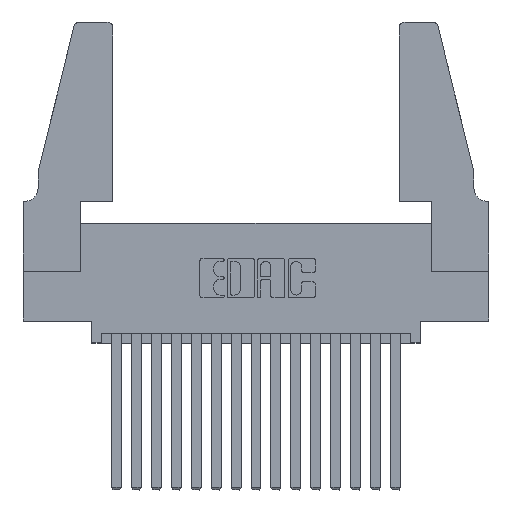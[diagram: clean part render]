
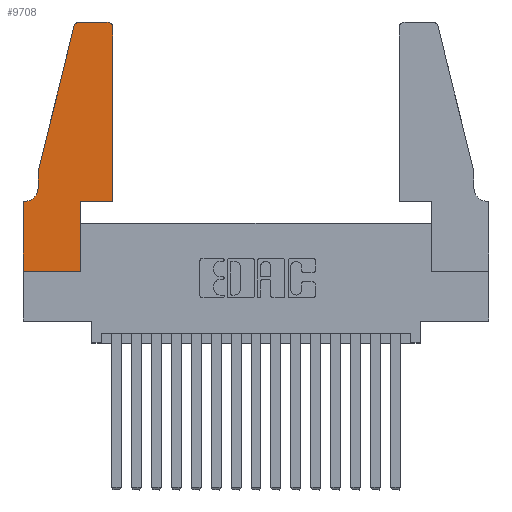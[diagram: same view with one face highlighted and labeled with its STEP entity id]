
A CAD part, top view. The second image highlights one B-rep face of the part: STEP entity #9708.
In plain terms, the highlighted planar face has unit normal (0, 0, 1).
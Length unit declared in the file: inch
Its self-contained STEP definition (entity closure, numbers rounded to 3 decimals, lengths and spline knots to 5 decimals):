
#396 = VECTOR ( 'NONE', #13454, 39.37008 ) ;
#656 = DIRECTION ( 'NONE',  ( 1., 0., 0. ) ) ;
#719 = VECTOR ( 'NONE', #10200, 39.37008 ) ;
#745 = PLANE ( 'NONE',  #5814 ) ;
#1059 = ORIENTED_EDGE ( 'NONE', *, *, #10012, .T. ) ;
#1159 = VERTEX_POINT ( 'NONE', #11331 ) ;
#1161 = LINE ( 'NONE', #16680, #719 ) ;
#1194 = LINE ( 'NONE', #2039, #4516 ) ;
#1454 = VERTEX_POINT ( 'NONE', #4281 ) ;
#1614 = VERTEX_POINT ( 'NONE', #7351 ) ;
#1761 = AXIS2_PLACEMENT_3D ( 'NONE', #14737, #6851, #16044 ) ;
#1959 = VECTOR ( 'NONE', #5132, 39.37008 ) ;
#2039 = CARTESIAN_POINT ( 'NONE',  ( 0.0755, 0.5, 0.37 ) ) ;
#2052 = LINE ( 'NONE', #10939, #9015 ) ;
#2414 = LINE ( 'NONE', #14403, #1959 ) ;
#2603 = EDGE_CURVE ( 'NONE', #14687, #13880, #5997, .T. ) ;
#2638 = CARTESIAN_POINT ( 'NONE',  ( 0.0755, 0.42, 0.37 ) ) ;
#3255 = AXIS2_PLACEMENT_3D ( 'NONE', #16836, #9037, #656 ) ;
#3266 = AXIS2_PLACEMENT_3D ( 'NONE', #7038, #16215, #8405 ) ;
#3308 = ORIENTED_EDGE ( 'NONE', *, *, #16690, .T. ) ;
#3374 = LINE ( 'NONE', #16887, #6653 ) ;
#3428 = VERTEX_POINT ( 'NONE', #11575 ) ;
#3618 = DIRECTION ( 'NONE',  ( 0., 0., 1. ) ) ;
#3692 = EDGE_CURVE ( 'NONE', #13880, #1159, #12225, .T. ) ;
#3773 = LINE ( 'NONE', #17414, #17524 ) ;
#4142 = DIRECTION ( 'NONE',  ( -1., 0., 0. ) ) ;
#4281 = CARTESIAN_POINT ( 'NONE',  ( 0., 0.35, 0.37 ) ) ;
#4516 = VECTOR ( 'NONE', #15460, 39.37008 ) ;
#5132 = DIRECTION ( 'NONE',  ( 0., 1., 0. ) ) ;
#5319 = VERTEX_POINT ( 'NONE', #12757 ) ;
#5472 = CARTESIAN_POINT ( 'NONE',  ( 0.2605, 1.25, 0.37 ) ) ;
#5486 = LINE ( 'NONE', #8207, #396 ) ;
#5509 = EDGE_CURVE ( 'NONE', #14080, #11525, #2414, .T. ) ;
#5814 = AXIS2_PLACEMENT_3D ( 'NONE', #11748, #3618, #13016 ) ;
#5864 = CARTESIAN_POINT ( 'NONE',  ( 0.0755, 0.5, 0.37 ) ) ;
#5997 = LINE ( 'NONE', #6854, #16541 ) ;
#6073 = VECTOR ( 'NONE', #12280, 39.37008 ) ;
#6595 = ORIENTED_EDGE ( 'NONE', *, *, #5509, .T. ) ;
#6653 = VECTOR ( 'NONE', #10412, 39.37008 ) ;
#6851 = DIRECTION ( 'NONE',  ( 0., 0., -1. ) ) ;
#6854 = CARTESIAN_POINT ( 'NONE',  ( 0.0755, 0.5, 0.37 ) ) ;
#7038 = CARTESIAN_POINT ( 'NONE',  ( 0.4205, 1.22, 0.37 ) ) ;
#7351 = CARTESIAN_POINT ( 'NONE',  ( 0.25487, 1.22718, 0.37 ) ) ;
#8207 = CARTESIAN_POINT ( 'NONE',  ( 0.4505, 0.35, 0.37 ) ) ;
#8274 = DIRECTION ( 'NONE',  ( 1., 0., 0. ) ) ;
#8376 = DIRECTION ( 'NONE',  ( 0., -1., 0. ) ) ;
#8405 = DIRECTION ( 'NONE',  ( 1., 0., 0. ) ) ;
#8479 = EDGE_CURVE ( 'NONE', #14214, #3428, #17027, .T. ) ;
#9015 = VECTOR ( 'NONE', #4142, 39.37008 ) ;
#9037 = DIRECTION ( 'NONE',  ( 0., 0., 1. ) ) ;
#9352 = ORIENTED_EDGE ( 'NONE', *, *, #9587, .T. ) ;
#9482 = VERTEX_POINT ( 'NONE', #14347 ) ;
#9537 = ORIENTED_EDGE ( 'NONE', *, *, #8479, .T. ) ;
#9587 = EDGE_CURVE ( 'NONE', #1454, #11561, #1161, .T. ) ;
#9708 = ADVANCED_FACE ( 'NONE', ( #16142 ), #745, .T. ) ;
#10012 = EDGE_CURVE ( 'NONE', #1159, #1454, #2052, .T. ) ;
#10200 = DIRECTION ( 'NONE',  ( 0., -1., 0. ) ) ;
#10270 = CARTESIAN_POINT ( 'NONE',  ( 0.2865, 0.35, 0.37 ) ) ;
#10324 = EDGE_CURVE ( 'NONE', #3428, #1614, #14487, .T. ) ;
#10359 = EDGE_CURVE ( 'NONE', #5319, #9482, #3374, .T. ) ;
#10381 = CARTESIAN_POINT ( 'NONE',  ( 0., 0., 0.37 ) ) ;
#10412 = DIRECTION ( 'NONE',  ( 0., 1., 0. ) ) ;
#10585 = ORIENTED_EDGE ( 'NONE', *, *, #10359, .T. ) ;
#10939 = CARTESIAN_POINT ( 'NONE',  ( 0.0755, 0.35, 0.37 ) ) ;
#11192 = ORIENTED_EDGE ( 'NONE', *, *, #13065, .T. ) ;
#11305 = CARTESIAN_POINT ( 'NONE',  ( 0.2865, 0., 0.37 ) ) ;
#11331 = CARTESIAN_POINT ( 'NONE',  ( 0.0055, 0.35, 0.37 ) ) ;
#11525 = VERTEX_POINT ( 'NONE', #10270 ) ;
#11561 = VERTEX_POINT ( 'NONE', #10381 ) ;
#11575 = CARTESIAN_POINT ( 'NONE',  ( 0.284, 1.25, 0.37 ) ) ;
#11748 = CARTESIAN_POINT ( 'NONE',  ( 0., 0.35, 0.37 ) ) ;
#11823 = EDGE_CURVE ( 'NONE', #11561, #14080, #3773, .T. ) ;
#12225 = CIRCLE ( 'NONE', #1761, 0.07 ) ;
#12280 = DIRECTION ( 'NONE',  ( -1., 0., 0. ) ) ;
#12757 = CARTESIAN_POINT ( 'NONE',  ( 0.4505, 0.35, 0.37 ) ) ;
#12797 = CIRCLE ( 'NONE', #3266, 0.03 ) ;
#13016 = DIRECTION ( 'NONE',  ( 1., 0., 0. ) ) ;
#13065 = EDGE_CURVE ( 'NONE', #1614, #14687, #1194, .T. ) ;
#13454 = DIRECTION ( 'NONE',  ( 1., 0., 0. ) ) ;
#13810 = ORIENTED_EDGE ( 'NONE', *, *, #10324, .T. ) ;
#13880 = VERTEX_POINT ( 'NONE', #2638 ) ;
#14080 = VERTEX_POINT ( 'NONE', #11305 ) ;
#14111 = CARTESIAN_POINT ( 'NONE',  ( 0.4205, 1.25, 0.37 ) ) ;
#14214 = VERTEX_POINT ( 'NONE', #14111 ) ;
#14347 = CARTESIAN_POINT ( 'NONE',  ( 0.4505, 1.22, 0.37 ) ) ;
#14403 = CARTESIAN_POINT ( 'NONE',  ( 0.2865, 0.35, 0.37 ) ) ;
#14487 = CIRCLE ( 'NONE', #3255, 0.03 ) ;
#14621 = ORIENTED_EDGE ( 'NONE', *, *, #2603, .T. ) ;
#14687 = VERTEX_POINT ( 'NONE', #5864 ) ;
#14737 = CARTESIAN_POINT ( 'NONE',  ( 0.0055, 0.42, 0.37 ) ) ;
#14843 = ORIENTED_EDGE ( 'NONE', *, *, #16102, .T. ) ;
#15039 = ORIENTED_EDGE ( 'NONE', *, *, #3692, .T. ) ;
#15460 = DIRECTION ( 'NONE',  ( -0.239, -0.971, 0. ) ) ;
#16044 = DIRECTION ( 'NONE',  ( -1., 0., 0. ) ) ;
#16102 = EDGE_CURVE ( 'NONE', #9482, #14214, #12797, .T. ) ;
#16142 = FACE_OUTER_BOUND ( 'NONE', #17133, .T. ) ;
#16215 = DIRECTION ( 'NONE',  ( 0., 0., 1. ) ) ;
#16541 = VECTOR ( 'NONE', #8376, 39.37008 ) ;
#16679 = ORIENTED_EDGE ( 'NONE', *, *, #11823, .T. ) ;
#16680 = CARTESIAN_POINT ( 'NONE',  ( 0., 0., 0.37 ) ) ;
#16690 = EDGE_CURVE ( 'NONE', #11525, #5319, #5486, .T. ) ;
#16836 = CARTESIAN_POINT ( 'NONE',  ( 0.284, 1.22, 0.37 ) ) ;
#16887 = CARTESIAN_POINT ( 'NONE',  ( 0.4505, 0.35, 0.37 ) ) ;
#17027 = LINE ( 'NONE', #5472, #6073 ) ;
#17133 = EDGE_LOOP ( 'NONE', ( #9537, #13810, #11192, #14621, #15039, #1059, #9352, #16679, #6595, #3308, #10585, #14843 ) ) ;
#17414 = CARTESIAN_POINT ( 'NONE',  ( 0., 0., 0.37 ) ) ;
#17524 = VECTOR ( 'NONE', #8274, 39.37008 ) ;
